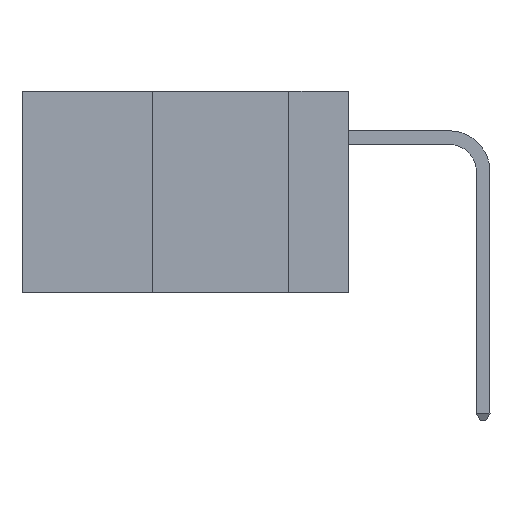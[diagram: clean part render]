
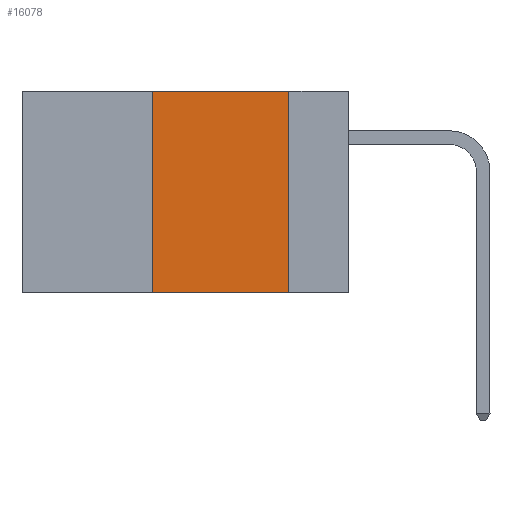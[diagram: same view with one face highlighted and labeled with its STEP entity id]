
A CAD part, left-side view. The second image highlights one B-rep face of the part: STEP entity #16078.
In plain terms, the highlighted planar face has unit normal (-1, 0, 0).
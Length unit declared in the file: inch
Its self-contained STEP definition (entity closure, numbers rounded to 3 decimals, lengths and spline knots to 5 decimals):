
#404 = DIRECTION ( 'NONE',  ( 1., 0., 0. ) ) ;
#2902 = EDGE_LOOP ( 'NONE', ( #26139, #5924, #6995, #17559 ) ) ;
#4974 = PLANE ( 'NONE',  #14084 ) ;
#5924 = ORIENTED_EDGE ( 'NONE', *, *, #20324, .F. ) ;
#6380 = VECTOR ( 'NONE', #6733, 39.37008 ) ;
#6733 = DIRECTION ( 'NONE',  ( 0., 0., -1. ) ) ;
#6995 = ORIENTED_EDGE ( 'NONE', *, *, #26054, .F. ) ;
#8109 = CARTESIAN_POINT ( 'NONE',  ( 0., 0.11, 0. ) ) ;
#9729 = CARTESIAN_POINT ( 'NONE',  ( 0., 0.36, 0. ) ) ;
#9732 = LINE ( 'NONE', #19318, #22053 ) ;
#10238 = VERTEX_POINT ( 'NONE', #30544 ) ;
#10823 = VECTOR ( 'NONE', #21198, 39.37008 ) ;
#12237 = LINE ( 'NONE', #19173, #10823 ) ;
#12335 = CARTESIAN_POINT ( 'NONE',  ( 0., 0.11, -0.37 ) ) ;
#13531 = VECTOR ( 'NONE', #29782, 39.37008 ) ;
#14084 = AXIS2_PLACEMENT_3D ( 'NONE', #24108, #404, #15178 ) ;
#15178 = DIRECTION ( 'NONE',  ( 0., 0., -1. ) ) ;
#16078 = ADVANCED_FACE ( 'NONE', ( #26455 ), #4974, .F. ) ;
#17476 = VERTEX_POINT ( 'NONE', #8109 ) ;
#17559 = ORIENTED_EDGE ( 'NONE', *, *, #18341, .T. ) ;
#18341 = EDGE_CURVE ( 'NONE', #10238, #24856, #22427, .T. ) ;
#19173 = CARTESIAN_POINT ( 'NONE',  ( 0., 0.36, 0. ) ) ;
#19318 = CARTESIAN_POINT ( 'NONE',  ( 0., 0.6, 0. ) ) ;
#20085 = CARTESIAN_POINT ( 'NONE',  ( 0., 0.6, -0.37 ) ) ;
#20324 = EDGE_CURVE ( 'NONE', #26184, #17476, #9732, .T. ) ;
#21198 = DIRECTION ( 'NONE',  ( 0., 0., 1. ) ) ;
#22053 = VECTOR ( 'NONE', #24154, 39.37008 ) ;
#22427 = LINE ( 'NONE', #20085, #13531 ) ;
#23832 = CARTESIAN_POINT ( 'NONE',  ( 0., 0.11, 0. ) ) ;
#24108 = CARTESIAN_POINT ( 'NONE',  ( 0., 0.6, 0. ) ) ;
#24154 = DIRECTION ( 'NONE',  ( 0., -1., 0. ) ) ;
#24856 = VERTEX_POINT ( 'NONE', #12335 ) ;
#26054 = EDGE_CURVE ( 'NONE', #10238, #26184, #12237, .T. ) ;
#26139 = ORIENTED_EDGE ( 'NONE', *, *, #27468, .F. ) ;
#26184 = VERTEX_POINT ( 'NONE', #9729 ) ;
#26455 = FACE_OUTER_BOUND ( 'NONE', #2902, .T. ) ;
#27468 = EDGE_CURVE ( 'NONE', #17476, #24856, #28231, .T. ) ;
#28231 = LINE ( 'NONE', #23832, #6380 ) ;
#29782 = DIRECTION ( 'NONE',  ( 0., -1., 0. ) ) ;
#30544 = CARTESIAN_POINT ( 'NONE',  ( 0., 0.36, -0.37 ) ) ;
